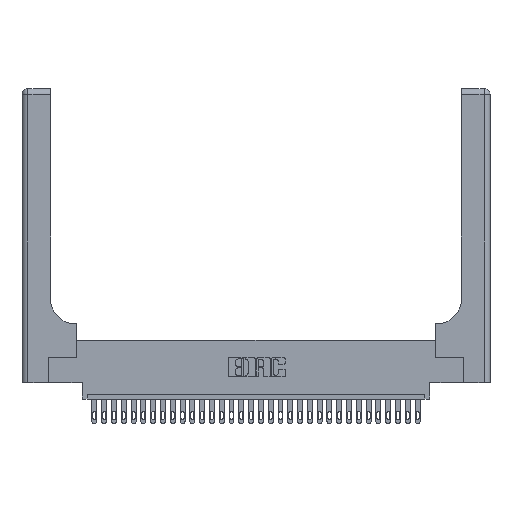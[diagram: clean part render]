
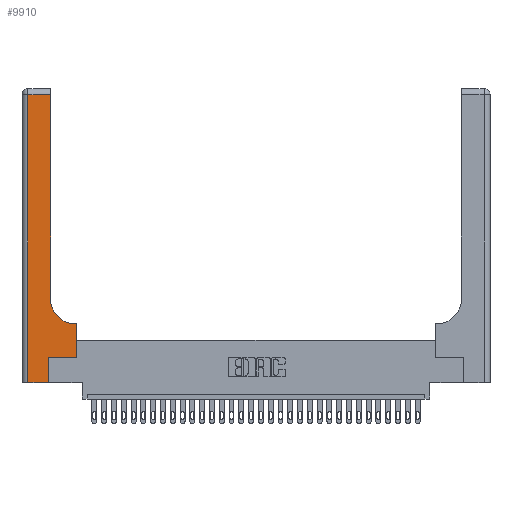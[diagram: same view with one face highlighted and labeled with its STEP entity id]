
A CAD part, top view. The second image highlights one B-rep face of the part: STEP entity #9910.
In plain terms, the highlighted planar face has unit normal (0, 0, 1).
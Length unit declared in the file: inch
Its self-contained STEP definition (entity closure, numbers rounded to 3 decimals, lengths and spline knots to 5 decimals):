
#114 = DIRECTION ( 'NONE',  ( 0., 1., 0. ) ) ;
#342 = ORIENTED_EDGE ( 'NONE', *, *, #12120, .T. ) ;
#557 = CARTESIAN_POINT ( 'NONE',  ( 0.06, 2.94, 0.37 ) ) ;
#1038 = LINE ( 'NONE', #11956, #14148 ) ;
#1621 = VECTOR ( 'NONE', #8458, 39.37008 ) ;
#2474 = VECTOR ( 'NONE', #23882, 39.37008 ) ;
#2497 = ORIENTED_EDGE ( 'NONE', *, *, #25977, .T. ) ;
#2564 = CARTESIAN_POINT ( 'NONE',  ( 0.5585, 0.25, 0.37 ) ) ;
#2717 = EDGE_CURVE ( 'NONE', #17322, #12620, #7775, .T. ) ;
#3199 = DIRECTION ( 'NONE',  ( 0., 0., -1. ) ) ;
#3863 = CARTESIAN_POINT ( 'NONE',  ( 0.269, 0., 0.37 ) ) ;
#3946 = CARTESIAN_POINT ( 'NONE',  ( 0.269, 0.25, 0.37 ) ) ;
#4443 = VERTEX_POINT ( 'NONE', #8573 ) ;
#4482 = CARTESIAN_POINT ( 'NONE',  ( 0.2915, 2.94, 0.37 ) ) ;
#4879 = EDGE_CURVE ( 'NONE', #12306, #17322, #31835, .T. ) ;
#5675 = VECTOR ( 'NONE', #17787, 39.37008 ) ;
#5984 = EDGE_CURVE ( 'NONE', #12620, #16816, #25988, .T. ) ;
#6214 = VERTEX_POINT ( 'NONE', #18280 ) ;
#7024 = CARTESIAN_POINT ( 'NONE',  ( 0.2915, 3., 0.37 ) ) ;
#7222 = LINE ( 'NONE', #15297, #5675 ) ;
#7353 = VECTOR ( 'NONE', #114, 39.37008 ) ;
#7775 = LINE ( 'NONE', #7024, #31286 ) ;
#8140 = ORIENTED_EDGE ( 'NONE', *, *, #28633, .T. ) ;
#8458 = DIRECTION ( 'NONE',  ( 0., 1., 0. ) ) ;
#8573 = CARTESIAN_POINT ( 'NONE',  ( 0.269, 0., 0.37 ) ) ;
#8812 = LINE ( 'NONE', #16788, #29632 ) ;
#9441 = DIRECTION ( 'NONE',  ( 1., 0., 0. ) ) ;
#9910 = ADVANCED_FACE ( 'NONE', ( #13004 ), #12680, .F. ) ;
#10737 = ORIENTED_EDGE ( 'NONE', *, *, #22106, .T. ) ;
#11956 = CARTESIAN_POINT ( 'NONE',  ( 0.269, 0.25, 0.37 ) ) ;
#12120 = EDGE_CURVE ( 'NONE', #22101, #4443, #8812, .T. ) ;
#12306 = VERTEX_POINT ( 'NONE', #14445 ) ;
#12620 = VERTEX_POINT ( 'NONE', #4482 ) ;
#12680 = PLANE ( 'NONE',  #24082 ) ;
#13004 = FACE_OUTER_BOUND ( 'NONE', #20800, .T. ) ;
#14148 = VECTOR ( 'NONE', #26977, 39.37008 ) ;
#14445 = CARTESIAN_POINT ( 'NONE',  ( 0.5415, 0.6, 0.37 ) ) ;
#15232 = DIRECTION ( 'NONE',  ( 1., 0., 0. ) ) ;
#15297 = CARTESIAN_POINT ( 'NONE',  ( 0.2915, 0.6, 0.37 ) ) ;
#15516 = AXIS2_PLACEMENT_3D ( 'NONE', #22581, #3199, #15232 ) ;
#15784 = CARTESIAN_POINT ( 'NONE',  ( 0.06, 3., 0.37 ) ) ;
#16118 = DIRECTION ( 'NONE',  ( 0., -1., 0. ) ) ;
#16355 = CARTESIAN_POINT ( 'NONE',  ( 0., 2.94, 0.37 ) ) ;
#16788 = CARTESIAN_POINT ( 'NONE',  ( 0., 0., 0.37 ) ) ;
#16816 = VERTEX_POINT ( 'NONE', #557 ) ;
#17322 = VERTEX_POINT ( 'NONE', #23579 ) ;
#17770 = VERTEX_POINT ( 'NONE', #2564 ) ;
#17787 = DIRECTION ( 'NONE',  ( -1., 0., 0. ) ) ;
#18280 = CARTESIAN_POINT ( 'NONE',  ( 0.5585, 0.6, 0.37 ) ) ;
#19650 = EDGE_CURVE ( 'NONE', #17770, #6214, #30446, .T. ) ;
#20039 = CARTESIAN_POINT ( 'NONE',  ( 0.5585, 0.25, 0.37 ) ) ;
#20800 = EDGE_LOOP ( 'NONE', ( #28427, #27854, #10737, #342, #2497, #21344, #25272, #8140, #23387 ) ) ;
#21344 = ORIENTED_EDGE ( 'NONE', *, *, #28448, .T. ) ;
#22101 = VERTEX_POINT ( 'NONE', #25810 ) ;
#22106 = EDGE_CURVE ( 'NONE', #16816, #22101, #27991, .T. ) ;
#22581 = CARTESIAN_POINT ( 'NONE',  ( 0.5415, 0.85, 0.37 ) ) ;
#22731 = DIRECTION ( 'NONE',  ( -1., 0., 0. ) ) ;
#23387 = ORIENTED_EDGE ( 'NONE', *, *, #4879, .T. ) ;
#23579 = CARTESIAN_POINT ( 'NONE',  ( 0.2915, 0.85, 0.37 ) ) ;
#23882 = DIRECTION ( 'NONE',  ( -1., 0., 0. ) ) ;
#24082 = AXIS2_PLACEMENT_3D ( 'NONE', #25104, #27582, #22731 ) ;
#24520 = VECTOR ( 'NONE', #16118, 39.37008 ) ;
#24785 = VERTEX_POINT ( 'NONE', #3946 ) ;
#25104 = CARTESIAN_POINT ( 'NONE',  ( 0., 3., 0.37 ) ) ;
#25272 = ORIENTED_EDGE ( 'NONE', *, *, #19650, .T. ) ;
#25474 = LINE ( 'NONE', #3863, #1621 ) ;
#25810 = CARTESIAN_POINT ( 'NONE',  ( 0.06, 0., 0.37 ) ) ;
#25977 = EDGE_CURVE ( 'NONE', #4443, #24785, #25474, .T. ) ;
#25988 = LINE ( 'NONE', #16355, #2474 ) ;
#26977 = DIRECTION ( 'NONE',  ( 1., 0., 0. ) ) ;
#27582 = DIRECTION ( 'NONE',  ( 0., 0., -1. ) ) ;
#27854 = ORIENTED_EDGE ( 'NONE', *, *, #5984, .T. ) ;
#27991 = LINE ( 'NONE', #15784, #24520 ) ;
#28427 = ORIENTED_EDGE ( 'NONE', *, *, #2717, .T. ) ;
#28448 = EDGE_CURVE ( 'NONE', #24785, #17770, #1038, .T. ) ;
#28633 = EDGE_CURVE ( 'NONE', #6214, #12306, #7222, .T. ) ;
#29220 = DIRECTION ( 'NONE',  ( 0., 1., 0. ) ) ;
#29632 = VECTOR ( 'NONE', #9441, 39.37008 ) ;
#30446 = LINE ( 'NONE', #20039, #7353 ) ;
#31286 = VECTOR ( 'NONE', #29220, 39.37008 ) ;
#31835 = CIRCLE ( 'NONE', #15516, 0.25 ) ;
